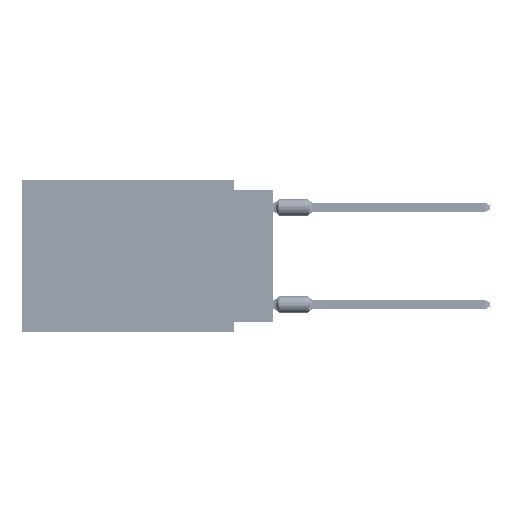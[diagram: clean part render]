
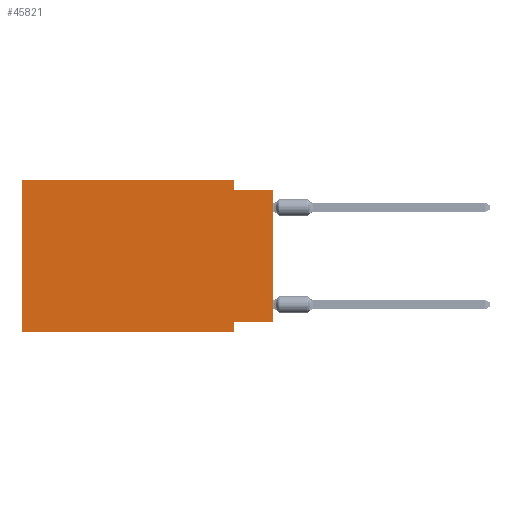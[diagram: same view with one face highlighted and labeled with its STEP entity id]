
A CAD part, left-side view. The second image highlights one B-rep face of the part: STEP entity #45821.
In plain terms, the highlighted planar face has unit normal (-1, 0, 0).
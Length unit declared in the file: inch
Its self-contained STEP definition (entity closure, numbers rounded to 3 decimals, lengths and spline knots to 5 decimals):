
#625 = LINE ( 'NONE', #59340, #31856 ) ;
#1854 = VECTOR ( 'NONE', #4628, 39.37008 ) ;
#4628 = DIRECTION ( 'NONE',  ( 0., -1., 0. ) ) ;
#4967 = CARTESIAN_POINT ( 'NONE',  ( 0., 0.645, 0. ) ) ;
#4972 = CARTESIAN_POINT ( 'NONE',  ( 0., 0.1, 0. ) ) ;
#5204 = VERTEX_POINT ( 'NONE', #74512 ) ;
#6955 = CARTESIAN_POINT ( 'NONE',  ( 0., 0.1, -0.39 ) ) ;
#9072 = VERTEX_POINT ( 'NONE', #6955 ) ;
#9361 = VERTEX_POINT ( 'NONE', #11738 ) ;
#11738 = CARTESIAN_POINT ( 'NONE',  ( 0., 0.1, -0.025 ) ) ;
#11986 = DIRECTION ( 'NONE',  ( 0., 0., 1. ) ) ;
#13293 = LINE ( 'NONE', #72450, #82876 ) ;
#13536 = VECTOR ( 'NONE', #41066, 39.37008 ) ;
#14707 = EDGE_CURVE ( 'NONE', #67131, #9361, #27117, .T. ) ;
#14766 = EDGE_CURVE ( 'NONE', #43392, #9072, #625, .T. ) ;
#16639 = ORIENTED_EDGE ( 'NONE', *, *, #66058, .F. ) ;
#18785 = DIRECTION ( 'NONE',  ( 1., 0., 0. ) ) ;
#19037 = VERTEX_POINT ( 'NONE', #53095 ) ;
#20737 = LINE ( 'NONE', #74585, #13536 ) ;
#22886 = ORIENTED_EDGE ( 'NONE', *, *, #56083, .T. ) ;
#24474 = CARTESIAN_POINT ( 'NONE',  ( 0., 0., -0.025 ) ) ;
#25567 = EDGE_LOOP ( 'NONE', ( #22886, #55831, #42161, #46918, #46974, #81761, #16639, #55785 ) ) ;
#27117 = LINE ( 'NONE', #39487, #37538 ) ;
#30200 = VECTOR ( 'NONE', #59529, 39.37008 ) ;
#31856 = VECTOR ( 'NONE', #86283, 39.37008 ) ;
#33730 = DIRECTION ( 'NONE',  ( 0., 0., -1. ) ) ;
#35251 = LINE ( 'NONE', #62169, #85240 ) ;
#35636 = CARTESIAN_POINT ( 'NONE',  ( 0., 0.645, -0.39 ) ) ;
#36543 = DIRECTION ( 'NONE',  ( 0., 0., -1. ) ) ;
#37538 = VECTOR ( 'NONE', #33730, 39.37008 ) ;
#38296 = EDGE_CURVE ( 'NONE', #43392, #59073, #20737, .T. ) ;
#38927 = LINE ( 'NONE', #81271, #76310 ) ;
#39487 = CARTESIAN_POINT ( 'NONE',  ( 0., 0.1, 0. ) ) ;
#41066 = DIRECTION ( 'NONE',  ( 0., 0., 1. ) ) ;
#42161 = ORIENTED_EDGE ( 'NONE', *, *, #14707, .F. ) ;
#43392 = VERTEX_POINT ( 'NONE', #35636 ) ;
#45305 = FACE_OUTER_BOUND ( 'NONE', #25567, .T. ) ;
#45723 = DIRECTION ( 'NONE',  ( 0., 0., -1. ) ) ;
#45821 = ADVANCED_FACE ( 'NONE', ( #45305 ), #52322, .F. ) ;
#46429 = AXIS2_PLACEMENT_3D ( 'NONE', #79264, #18785, #45723 ) ;
#46918 = ORIENTED_EDGE ( 'NONE', *, *, #47911, .F. ) ;
#46974 = ORIENTED_EDGE ( 'NONE', *, *, #38296, .F. ) ;
#47911 = EDGE_CURVE ( 'NONE', #59073, #67131, #38927, .T. ) ;
#51345 = VERTEX_POINT ( 'NONE', #56883 ) ;
#52322 = PLANE ( 'NONE',  #46429 ) ;
#53095 = CARTESIAN_POINT ( 'NONE',  ( 0., 0., -0.025 ) ) ;
#55785 = ORIENTED_EDGE ( 'NONE', *, *, #78885, .F. ) ;
#55831 = ORIENTED_EDGE ( 'NONE', *, *, #86455, .F. ) ;
#56083 = EDGE_CURVE ( 'NONE', #51345, #19037, #13293, .T. ) ;
#56883 = CARTESIAN_POINT ( 'NONE',  ( 0., 0., -0.365 ) ) ;
#59073 = VERTEX_POINT ( 'NONE', #4967 ) ;
#59195 = DIRECTION ( 'NONE',  ( 0., -1., 0. ) ) ;
#59340 = CARTESIAN_POINT ( 'NONE',  ( 0., 0.645, -0.39 ) ) ;
#59529 = DIRECTION ( 'NONE',  ( 0., 1., 0. ) ) ;
#62169 = CARTESIAN_POINT ( 'NONE',  ( 0., 0.1, -0.39 ) ) ;
#66058 = EDGE_CURVE ( 'NONE', #5204, #9072, #35251, .T. ) ;
#67131 = VERTEX_POINT ( 'NONE', #4972 ) ;
#71271 = LINE ( 'NONE', #24474, #1854 ) ;
#72450 = CARTESIAN_POINT ( 'NONE',  ( 0., 0., 0. ) ) ;
#73202 = CARTESIAN_POINT ( 'NONE',  ( 0., 0., -0.365 ) ) ;
#74512 = CARTESIAN_POINT ( 'NONE',  ( 0., 0.1, -0.365 ) ) ;
#74585 = CARTESIAN_POINT ( 'NONE',  ( 0., 0.645, 0. ) ) ;
#76310 = VECTOR ( 'NONE', #59195, 39.37008 ) ;
#78885 = EDGE_CURVE ( 'NONE', #51345, #5204, #86462, .T. ) ;
#79264 = CARTESIAN_POINT ( 'NONE',  ( 0., 0.645, 0. ) ) ;
#81271 = CARTESIAN_POINT ( 'NONE',  ( 0., 0.645, 0. ) ) ;
#81761 = ORIENTED_EDGE ( 'NONE', *, *, #14766, .T. ) ;
#82876 = VECTOR ( 'NONE', #11986, 39.37008 ) ;
#85240 = VECTOR ( 'NONE', #36543, 39.37008 ) ;
#86283 = DIRECTION ( 'NONE',  ( 0., -1., 0. ) ) ;
#86455 = EDGE_CURVE ( 'NONE', #9361, #19037, #71271, .T. ) ;
#86462 = LINE ( 'NONE', #73202, #30200 ) ;
